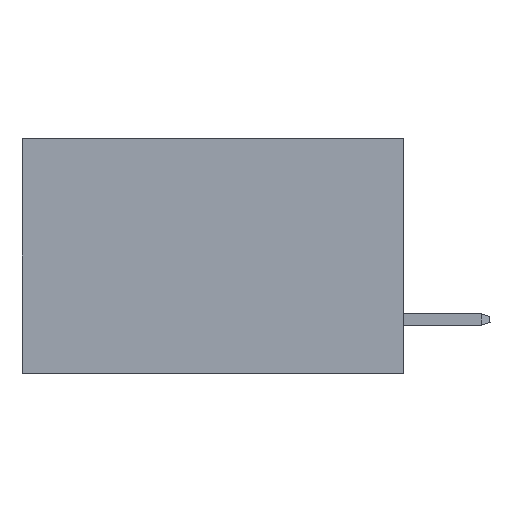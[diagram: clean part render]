
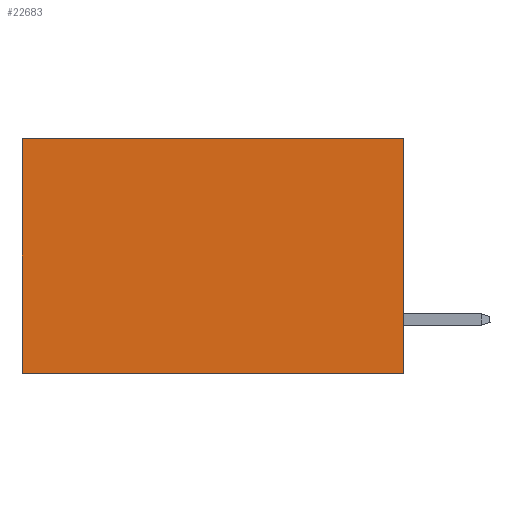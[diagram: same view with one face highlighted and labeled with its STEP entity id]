
A CAD part, left-side view. The second image highlights one B-rep face of the part: STEP entity #22683.
In plain terms, the highlighted planar face has unit normal (-1, 0, 0).
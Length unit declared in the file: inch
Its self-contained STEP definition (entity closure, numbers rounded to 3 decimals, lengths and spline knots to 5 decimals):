
#268 = DIRECTION ( 'NONE',  ( 0., 1., 0. ) ) ;
#311 = CARTESIAN_POINT ( 'NONE',  ( 0.2875, 0., -0.37 ) ) ;
#433 = EDGE_CURVE ( 'NONE', #3248, #2647, #8078, .T. ) ;
#1151 = VECTOR ( 'NONE', #5830, 39.37008 ) ;
#1967 = CARTESIAN_POINT ( 'NONE',  ( 0.2875, 0.6, 0. ) ) ;
#2647 = VERTEX_POINT ( 'NONE', #19259 ) ;
#3248 = VERTEX_POINT ( 'NONE', #1967 ) ;
#3953 = PLANE ( 'NONE',  #9285 ) ;
#4194 = DIRECTION ( 'NONE',  ( 0., 0., -1. ) ) ;
#5561 = EDGE_CURVE ( 'NONE', #11957, #2647, #20359, .T. ) ;
#5830 = DIRECTION ( 'NONE',  ( 0., 1., 0. ) ) ;
#6790 = LINE ( 'NONE', #18487, #1151 ) ;
#6994 = DIRECTION ( 'NONE',  ( 0., 0., -1. ) ) ;
#7512 = FACE_OUTER_BOUND ( 'NONE', #19945, .T. ) ;
#8078 = LINE ( 'NONE', #11731, #22851 ) ;
#9277 = VECTOR ( 'NONE', #268, 39.37008 ) ;
#9285 = AXIS2_PLACEMENT_3D ( 'NONE', #13285, #13055, #4194 ) ;
#9365 = CARTESIAN_POINT ( 'NONE',  ( 0.2875, 0., -0.37 ) ) ;
#10196 = DIRECTION ( 'NONE',  ( 0., 0., -1. ) ) ;
#11297 = CARTESIAN_POINT ( 'NONE',  ( 0.2875, 0., 0. ) ) ;
#11731 = CARTESIAN_POINT ( 'NONE',  ( 0.2875, 0.6, 0. ) ) ;
#11957 = VERTEX_POINT ( 'NONE', #311 ) ;
#12289 = EDGE_CURVE ( 'NONE', #18523, #3248, #6790, .T. ) ;
#12351 = ORIENTED_EDGE ( 'NONE', *, *, #433, .T. ) ;
#13055 = DIRECTION ( 'NONE',  ( 1., 0., 0. ) ) ;
#13285 = CARTESIAN_POINT ( 'NONE',  ( 0.2875, 0., 0. ) ) ;
#13886 = EDGE_CURVE ( 'NONE', #18523, #11957, #22982, .T. ) ;
#17043 = VECTOR ( 'NONE', #6994, 39.37008 ) ;
#18487 = CARTESIAN_POINT ( 'NONE',  ( 0.2875, 0., 0. ) ) ;
#18523 = VERTEX_POINT ( 'NONE', #11297 ) ;
#18712 = ORIENTED_EDGE ( 'NONE', *, *, #5561, .F. ) ;
#19259 = CARTESIAN_POINT ( 'NONE',  ( 0.2875, 0.6, -0.37 ) ) ;
#19945 = EDGE_LOOP ( 'NONE', ( #12351, #18712, #20265, #21530 ) ) ;
#20265 = ORIENTED_EDGE ( 'NONE', *, *, #13886, .F. ) ;
#20359 = LINE ( 'NONE', #9365, #9277 ) ;
#21530 = ORIENTED_EDGE ( 'NONE', *, *, #12289, .T. ) ;
#22683 = ADVANCED_FACE ( 'NONE', ( #7512 ), #3953, .F. ) ;
#22851 = VECTOR ( 'NONE', #10196, 39.37008 ) ;
#22982 = LINE ( 'NONE', #23213, #17043 ) ;
#23213 = CARTESIAN_POINT ( 'NONE',  ( 0.2875, 0., 0. ) ) ;
